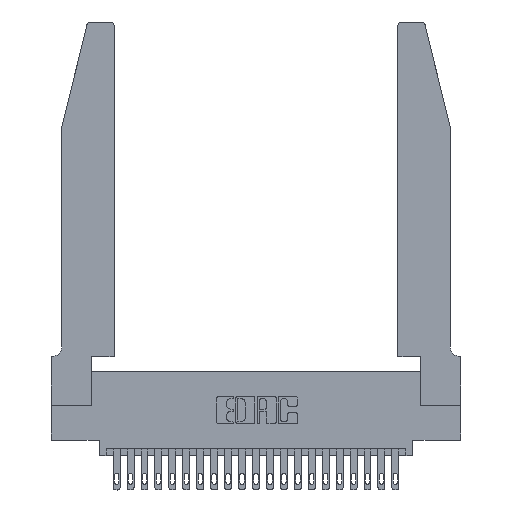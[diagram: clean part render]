
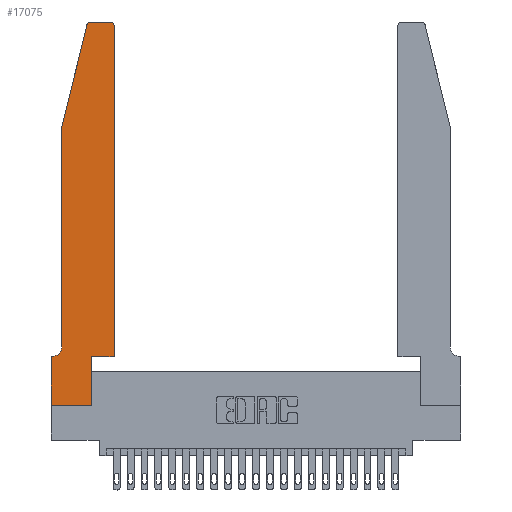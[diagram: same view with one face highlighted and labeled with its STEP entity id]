
A CAD part, top view. The second image highlights one B-rep face of the part: STEP entity #17075.
In plain terms, the highlighted planar face has unit normal (0, 0, 1).
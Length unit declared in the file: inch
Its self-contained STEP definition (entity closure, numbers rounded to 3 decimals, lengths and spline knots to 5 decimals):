
#214 = EDGE_CURVE ( 'NONE', #9538, #20990, #14880, .T. ) ;
#221 = CARTESIAN_POINT ( 'NONE',  ( 0.0055, 0.42, 0.37 ) ) ;
#244 = LINE ( 'NONE', #14087, #12548 ) ;
#454 = DIRECTION ( 'NONE',  ( 0., 1., 0. ) ) ;
#485 = CARTESIAN_POINT ( 'NONE',  ( 0.2865, 0.35, 0.37 ) ) ;
#514 = VECTOR ( 'NONE', #11498, 39.37008 ) ;
#738 = CARTESIAN_POINT ( 'NONE',  ( 0.0755, 2., 0.37 ) ) ;
#841 = CARTESIAN_POINT ( 'NONE',  ( 0.4505, 0.35, 0.37 ) ) ;
#1118 = EDGE_CURVE ( 'NONE', #7602, #7371, #13951, .T. ) ;
#1334 = AXIS2_PLACEMENT_3D ( 'NONE', #5428, #8893, #14517 ) ;
#1373 = EDGE_CURVE ( 'NONE', #8115, #9538, #21167, .T. ) ;
#1519 = VERTEX_POINT ( 'NONE', #22447 ) ;
#2113 = CARTESIAN_POINT ( 'NONE',  ( 0.0755, 0.35, 0.37 ) ) ;
#2374 = ORIENTED_EDGE ( 'NONE', *, *, #1373, .T. ) ;
#3005 = CIRCLE ( 'NONE', #9562, 0.03 ) ;
#3047 = DIRECTION ( 'NONE',  ( -1., 0., 0. ) ) ;
#3078 = ORIENTED_EDGE ( 'NONE', *, *, #214, .T. ) ;
#3223 = VECTOR ( 'NONE', #20169, 39.37008 ) ;
#3619 = CARTESIAN_POINT ( 'NONE',  ( 0.4205, 2.72, 0.37 ) ) ;
#4658 = DIRECTION ( 'NONE',  ( 1., 0., 0. ) ) ;
#4763 = CARTESIAN_POINT ( 'NONE',  ( 0.4505, 2.72, 0.37 ) ) ;
#5077 = EDGE_CURVE ( 'NONE', #17762, #7602, #16814, .T. ) ;
#5428 = CARTESIAN_POINT ( 'NONE',  ( 0.284, 2.72, 0.37 ) ) ;
#5522 = DIRECTION ( 'NONE',  ( -0.239, -0.971, 0. ) ) ;
#5638 = FACE_OUTER_BOUND ( 'NONE', #11593, .T. ) ;
#5844 = VERTEX_POINT ( 'NONE', #9144 ) ;
#6843 = VERTEX_POINT ( 'NONE', #17821 ) ;
#7022 = CARTESIAN_POINT ( 'NONE',  ( 0.2605, 2.75, 0.37 ) ) ;
#7321 = CARTESIAN_POINT ( 'NONE',  ( 0.0055, 0.35, 0.37 ) ) ;
#7371 = VERTEX_POINT ( 'NONE', #4763 ) ;
#7602 = VERTEX_POINT ( 'NONE', #10610 ) ;
#7629 = ORIENTED_EDGE ( 'NONE', *, *, #5077, .T. ) ;
#7756 = DIRECTION ( 'NONE',  ( -1., 0., 0. ) ) ;
#7856 = VECTOR ( 'NONE', #454, 39.37008 ) ;
#8115 = VERTEX_POINT ( 'NONE', #738 ) ;
#8893 = DIRECTION ( 'NONE',  ( 0., 0., 1. ) ) ;
#8970 = ORIENTED_EDGE ( 'NONE', *, *, #9804, .T. ) ;
#8971 = DIRECTION ( 'NONE',  ( 0., 0., 1. ) ) ;
#9144 = CARTESIAN_POINT ( 'NONE',  ( 0., 0., 0.37 ) ) ;
#9154 = EDGE_CURVE ( 'NONE', #21474, #8115, #14651, .T. ) ;
#9212 = ORIENTED_EDGE ( 'NONE', *, *, #10105, .T. ) ;
#9251 = CIRCLE ( 'NONE', #1334, 0.03 ) ;
#9295 = DIRECTION ( 'NONE',  ( 0., 0., -1. ) ) ;
#9538 = VERTEX_POINT ( 'NONE', #21274 ) ;
#9562 = AXIS2_PLACEMENT_3D ( 'NONE', #3619, #8971, #10978 ) ;
#9804 = EDGE_CURVE ( 'NONE', #17250, #5844, #244, .T. ) ;
#9856 = ORIENTED_EDGE ( 'NONE', *, *, #22640, .T. ) ;
#9936 = ORIENTED_EDGE ( 'NONE', *, *, #1118, .T. ) ;
#10105 = EDGE_CURVE ( 'NONE', #7371, #20304, #3005, .T. ) ;
#10269 = CARTESIAN_POINT ( 'NONE',  ( 0., 0.35, 0.37 ) ) ;
#10314 = DIRECTION ( 'NONE',  ( 0., -1., 0. ) ) ;
#10468 = LINE ( 'NONE', #485, #514 ) ;
#10610 = CARTESIAN_POINT ( 'NONE',  ( 0.4505, 0.35, 0.37 ) ) ;
#10630 = LINE ( 'NONE', #2113, #17318 ) ;
#10978 = DIRECTION ( 'NONE',  ( 1., 0., 0. ) ) ;
#11008 = EDGE_CURVE ( 'NONE', #5844, #1519, #13674, .T. ) ;
#11430 = EDGE_CURVE ( 'NONE', #1519, #17762, #10468, .T. ) ;
#11454 = VECTOR ( 'NONE', #3047, 39.37008 ) ;
#11498 = DIRECTION ( 'NONE',  ( 0., 1., 0. ) ) ;
#11593 = EDGE_LOOP ( 'NONE', ( #9856, #22894, #15104, #2374, #3078, #23798, #8970, #13940, #13215, #7629, #9936, #9212 ) ) ;
#12119 = AXIS2_PLACEMENT_3D ( 'NONE', #221, #9295, #23963 ) ;
#12214 = PLANE ( 'NONE',  #13219 ) ;
#12548 = VECTOR ( 'NONE', #10314, 39.37008 ) ;
#12575 = VECTOR ( 'NONE', #5522, 39.37008 ) ;
#13077 = CARTESIAN_POINT ( 'NONE',  ( 0., 0., 0.37 ) ) ;
#13215 = ORIENTED_EDGE ( 'NONE', *, *, #11430, .T. ) ;
#13219 = AXIS2_PLACEMENT_3D ( 'NONE', #10269, #19521, #23042 ) ;
#13674 = LINE ( 'NONE', #13077, #20914 ) ;
#13940 = ORIENTED_EDGE ( 'NONE', *, *, #11008, .T. ) ;
#13951 = LINE ( 'NONE', #17192, #7856 ) ;
#14060 = CARTESIAN_POINT ( 'NONE',  ( 0.2865, 0.35, 0.37 ) ) ;
#14087 = CARTESIAN_POINT ( 'NONE',  ( 0., 0., 0.37 ) ) ;
#14517 = DIRECTION ( 'NONE',  ( 1., 0., 0. ) ) ;
#14651 = LINE ( 'NONE', #23545, #12575 ) ;
#14696 = CARTESIAN_POINT ( 'NONE',  ( 0.0755, 2., 0.37 ) ) ;
#14880 = CIRCLE ( 'NONE', #12119, 0.07 ) ;
#14968 = DIRECTION ( 'NONE',  ( 1., 0., 0. ) ) ;
#15104 = ORIENTED_EDGE ( 'NONE', *, *, #9154, .T. ) ;
#15839 = EDGE_CURVE ( 'NONE', #20990, #17250, #10630, .T. ) ;
#16532 = CARTESIAN_POINT ( 'NONE',  ( 0.4205, 2.75, 0.37 ) ) ;
#16814 = LINE ( 'NONE', #841, #23794 ) ;
#17075 = ADVANCED_FACE ( 'NONE', ( #5638 ), #12214, .T. ) ;
#17192 = CARTESIAN_POINT ( 'NONE',  ( 0.4505, 0.35, 0.37 ) ) ;
#17250 = VERTEX_POINT ( 'NONE', #20012 ) ;
#17318 = VECTOR ( 'NONE', #7756, 39.37008 ) ;
#17762 = VERTEX_POINT ( 'NONE', #14060 ) ;
#17821 = CARTESIAN_POINT ( 'NONE',  ( 0.284, 2.75, 0.37 ) ) ;
#19521 = DIRECTION ( 'NONE',  ( 0., 0., 1. ) ) ;
#19625 = CARTESIAN_POINT ( 'NONE',  ( 0.25487, 2.72718, 0.37 ) ) ;
#20012 = CARTESIAN_POINT ( 'NONE',  ( 0., 0.35, 0.37 ) ) ;
#20169 = DIRECTION ( 'NONE',  ( 0., -1., 0. ) ) ;
#20304 = VERTEX_POINT ( 'NONE', #16532 ) ;
#20338 = EDGE_CURVE ( 'NONE', #6843, #21474, #9251, .T. ) ;
#20914 = VECTOR ( 'NONE', #14968, 39.37008 ) ;
#20990 = VERTEX_POINT ( 'NONE', #7321 ) ;
#21167 = LINE ( 'NONE', #14696, #3223 ) ;
#21274 = CARTESIAN_POINT ( 'NONE',  ( 0.0755, 0.42, 0.37 ) ) ;
#21474 = VERTEX_POINT ( 'NONE', #19625 ) ;
#21966 = LINE ( 'NONE', #7022, #11454 ) ;
#22447 = CARTESIAN_POINT ( 'NONE',  ( 0.2865, 0., 0.37 ) ) ;
#22640 = EDGE_CURVE ( 'NONE', #20304, #6843, #21966, .T. ) ;
#22894 = ORIENTED_EDGE ( 'NONE', *, *, #20338, .T. ) ;
#23042 = DIRECTION ( 'NONE',  ( 1., 0., 0. ) ) ;
#23545 = CARTESIAN_POINT ( 'NONE',  ( 0.0755, 2., 0.37 ) ) ;
#23794 = VECTOR ( 'NONE', #4658, 39.37008 ) ;
#23798 = ORIENTED_EDGE ( 'NONE', *, *, #15839, .T. ) ;
#23963 = DIRECTION ( 'NONE',  ( -1., 0., 0. ) ) ;
